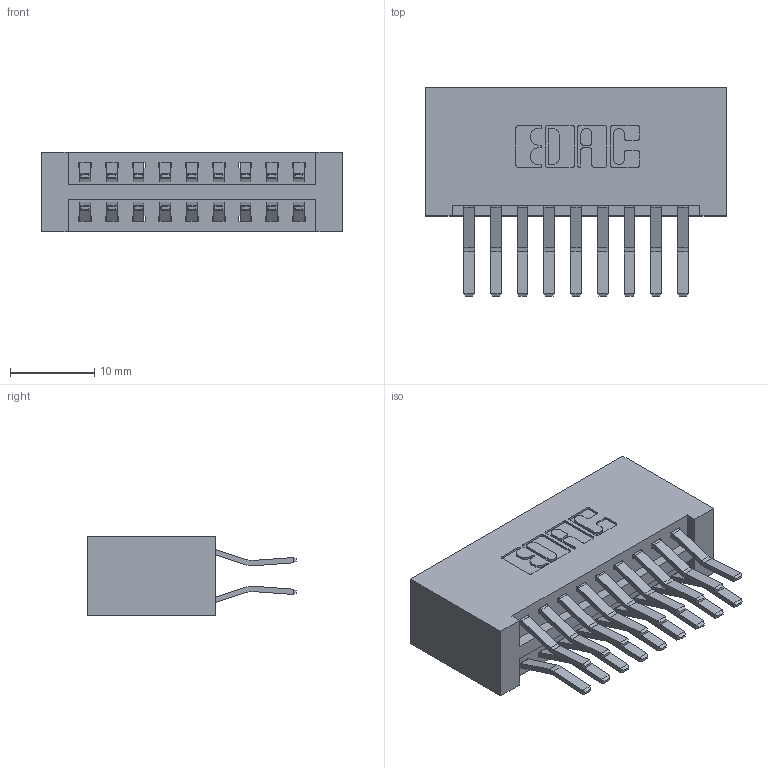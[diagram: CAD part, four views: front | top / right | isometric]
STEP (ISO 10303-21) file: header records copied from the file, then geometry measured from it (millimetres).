
FILE_DESCRIPTION (( 'STEP AP203' ), '1' );
FILE_NAME ('346-018-560-201.STEP', '2022-05-18T18:19:37', ( '' ), ( '' ), 'SwSTEP 2.0', 'SolidWorks 2020', '' );
FILE_SCHEMA (( 'CONFIG_CONTROL_DESIGN' ));
Length unit declared in the file: inch
Products named in the file (3): 345-292-001_560 Tail; 346-018-560-201; 346 Part_No Mounting Lugs
Assembly tree (19 placements, depth 2):
  346-018-560-201
    346 Part_No Mounting Lugs
    345-292-001_560 Tail  x18
Bounding box: 35.81 x 24.78 x 9.4 mm (x, y, z)
Volume: 3927.3 mm3; surface area: 5357.6 mm2
Topology: 19 solids, 19 shells, 1086 faces, 3203 edges, 2110 vertices
Faces by surface type: plane 702, cylinder 384
Entity records: 10127 total; most frequent: CARTESIAN_POINT 1712, ORIENTED_EDGE 1646, DIRECTION 1559, EDGE_CURVE 823, LINE 659, VECTOR 659, VERTEX_POINT 546, AXIS2_PLACEMENT_3D 450
